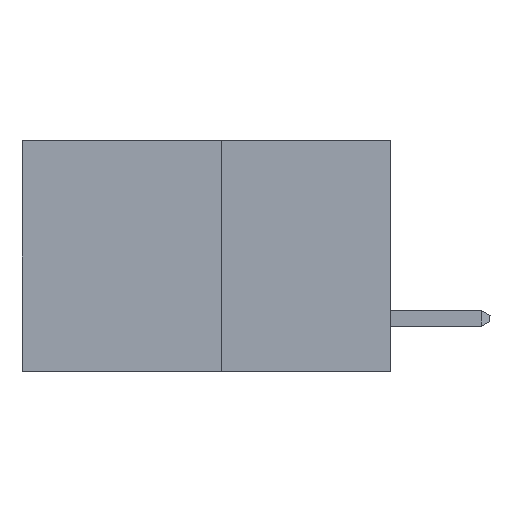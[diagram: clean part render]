
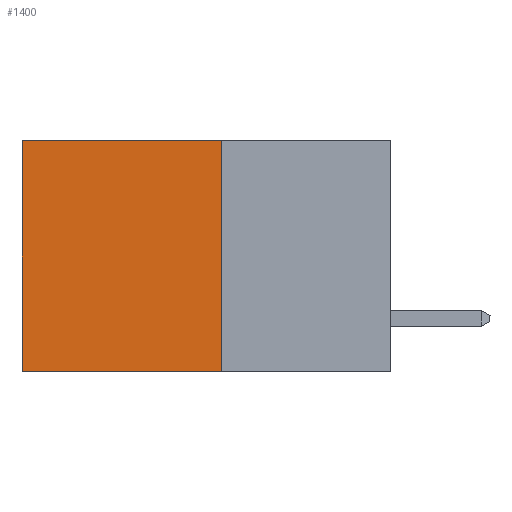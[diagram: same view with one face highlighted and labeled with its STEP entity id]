
A CAD part, left-side view. The second image highlights one B-rep face of the part: STEP entity #1400.
In plain terms, the highlighted planar face has unit normal (-1, 0, 0).
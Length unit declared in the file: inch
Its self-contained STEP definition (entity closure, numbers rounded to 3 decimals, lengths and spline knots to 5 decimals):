
#74 = CARTESIAN_POINT ( 'NONE',  ( 0.277, 0.27, -0.37 ) ) ;
#693 = VERTEX_POINT ( 'NONE', #6940 ) ;
#1400 = ADVANCED_FACE ( 'NONE', ( #3401 ), #5648, .F. ) ;
#1488 = ORIENTED_EDGE ( 'NONE', *, *, #8778, .T. ) ;
#1744 = LINE ( 'NONE', #3140, #1980 ) ;
#1843 = LINE ( 'NONE', #2279, #3707 ) ;
#1980 = VECTOR ( 'NONE', #8710, 39.37008 ) ;
#2279 = CARTESIAN_POINT ( 'NONE',  ( 0.277, 0.27, 0. ) ) ;
#2308 = DIRECTION ( 'NONE',  ( 0., 1., 0. ) ) ;
#2321 = DIRECTION ( 'NONE',  ( 0., 1., 0. ) ) ;
#2816 = CARTESIAN_POINT ( 'NONE',  ( 0.277, 0.27, -0.37 ) ) ;
#2849 = EDGE_CURVE ( 'NONE', #7862, #5149, #8240, .T. ) ;
#3070 = EDGE_LOOP ( 'NONE', ( #1488, #4561, #4206, #9729 ) ) ;
#3134 = EDGE_CURVE ( 'NONE', #693, #6852, #1843, .T. ) ;
#3140 = CARTESIAN_POINT ( 'NONE',  ( 0.277, 0.59, -0.37 ) ) ;
#3401 = FACE_OUTER_BOUND ( 'NONE', #3070, .T. ) ;
#3625 = EDGE_CURVE ( 'NONE', #693, #7862, #7704, .T. ) ;
#3707 = VECTOR ( 'NONE', #2321, 39.37008 ) ;
#3710 = CARTESIAN_POINT ( 'NONE',  ( 0.277, 0.27, -0.37 ) ) ;
#4206 = ORIENTED_EDGE ( 'NONE', *, *, #3625, .F. ) ;
#4561 = ORIENTED_EDGE ( 'NONE', *, *, #2849, .F. ) ;
#4796 = CARTESIAN_POINT ( 'NONE',  ( 0.277, 0.59, 0. ) ) ;
#5149 = VERTEX_POINT ( 'NONE', #8123 ) ;
#5264 = AXIS2_PLACEMENT_3D ( 'NONE', #7696, #6465, #5778 ) ;
#5565 = VECTOR ( 'NONE', #9255, 39.37008 ) ;
#5648 = PLANE ( 'NONE',  #5264 ) ;
#5778 = DIRECTION ( 'NONE',  ( 0., 0., -1. ) ) ;
#6465 = DIRECTION ( 'NONE',  ( 1., 0., 0. ) ) ;
#6621 = VECTOR ( 'NONE', #2308, 39.37008 ) ;
#6852 = VERTEX_POINT ( 'NONE', #4796 ) ;
#6940 = CARTESIAN_POINT ( 'NONE',  ( 0.277, 0.27, 0. ) ) ;
#7696 = CARTESIAN_POINT ( 'NONE',  ( 0.277, 0.27, -0.37 ) ) ;
#7704 = LINE ( 'NONE', #3710, #5565 ) ;
#7862 = VERTEX_POINT ( 'NONE', #2816 ) ;
#8123 = CARTESIAN_POINT ( 'NONE',  ( 0.277, 0.59, -0.37 ) ) ;
#8240 = LINE ( 'NONE', #74, #6621 ) ;
#8710 = DIRECTION ( 'NONE',  ( 0., 0., -1. ) ) ;
#8778 = EDGE_CURVE ( 'NONE', #6852, #5149, #1744, .T. ) ;
#9255 = DIRECTION ( 'NONE',  ( 0., 0., -1. ) ) ;
#9729 = ORIENTED_EDGE ( 'NONE', *, *, #3134, .T. ) ;
